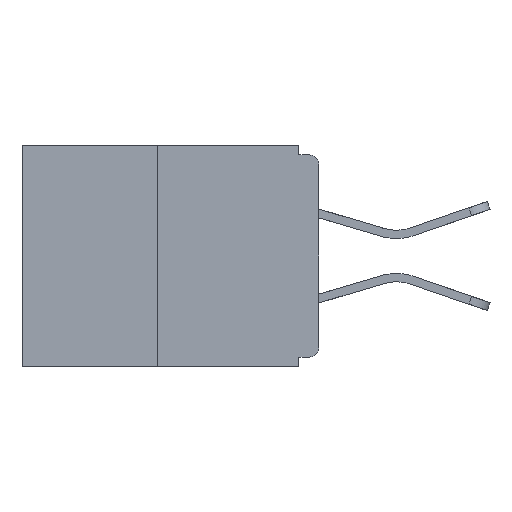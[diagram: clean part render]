
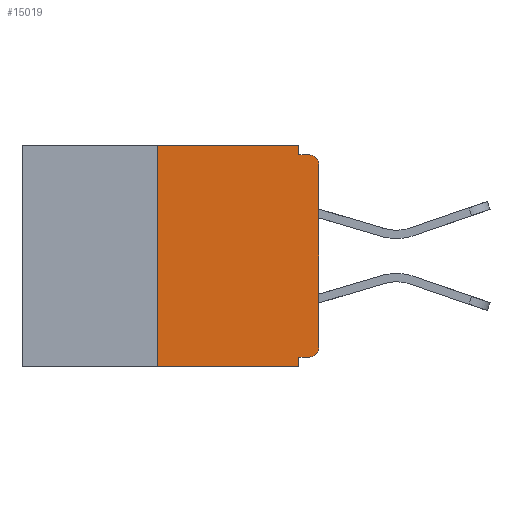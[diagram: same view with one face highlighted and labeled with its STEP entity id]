
A CAD part, left-side view. The second image highlights one B-rep face of the part: STEP entity #15019.
In plain terms, the highlighted planar face has unit normal (-1, 0, 0).
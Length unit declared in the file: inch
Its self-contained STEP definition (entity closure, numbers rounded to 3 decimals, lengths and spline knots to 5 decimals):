
#645 = VERTEX_POINT ( 'NONE', #8346 ) ;
#1054 = VERTEX_POINT ( 'NONE', #18536 ) ;
#2759 = CARTESIAN_POINT ( 'NONE',  ( 0., 0., -0.313 ) ) ;
#2954 = VERTEX_POINT ( 'NONE', #23299 ) ;
#3168 = LINE ( 'NONE', #16092, #10694 ) ;
#3384 = LINE ( 'NONE', #19765, #8680 ) ;
#4042 = ORIENTED_EDGE ( 'NONE', *, *, #25204, .F. ) ;
#4193 = LINE ( 'NONE', #7287, #13943 ) ;
#4215 = EDGE_LOOP ( 'NONE', ( #4042, #20265, #28305, #14607, #9492, #30821, #9199, #12878, #24777, #8813 ) ) ;
#4733 = CARTESIAN_POINT ( 'NONE',  ( 0., 0.015, -0.328 ) ) ;
#4757 = FACE_OUTER_BOUND ( 'NONE', #4215, .T. ) ;
#5252 = CARTESIAN_POINT ( 'NONE',  ( 0., 0., 0. ) ) ;
#5869 = CARTESIAN_POINT ( 'NONE',  ( 0., 0.015, -0.03 ) ) ;
#5882 = CARTESIAN_POINT ( 'NONE',  ( 0., 0.015, -0.313 ) ) ;
#5987 = DIRECTION ( 'NONE',  ( 0., 0., -1. ) ) ;
#6419 = EDGE_CURVE ( 'NONE', #29042, #29580, #3384, .T. ) ;
#6627 = EDGE_CURVE ( 'NONE', #20547, #26070, #18363, .T. ) ;
#6712 = CARTESIAN_POINT ( 'NONE',  ( 0., 0.031, -0.328 ) ) ;
#6923 = CARTESIAN_POINT ( 'NONE',  ( 0., 0.031, 0. ) ) ;
#7287 = CARTESIAN_POINT ( 'NONE',  ( 0., 0.46, -0.343 ) ) ;
#7476 = DIRECTION ( 'NONE',  ( 0., 0., -1. ) ) ;
#8002 = CIRCLE ( 'NONE', #30102, 0.015 ) ;
#8346 = CARTESIAN_POINT ( 'NONE',  ( 0., 0., -0.03 ) ) ;
#8675 = DIRECTION ( 'NONE',  ( 0., 0., 1. ) ) ;
#8680 = VECTOR ( 'NONE', #7476, 39.37008 ) ;
#8813 = ORIENTED_EDGE ( 'NONE', *, *, #6419, .F. ) ;
#8964 = CARTESIAN_POINT ( 'NONE',  ( 0., 0.031, -0.343 ) ) ;
#9162 = EDGE_CURVE ( 'NONE', #29580, #1054, #24224, .T. ) ;
#9199 = ORIENTED_EDGE ( 'NONE', *, *, #20793, .T. ) ;
#9492 = ORIENTED_EDGE ( 'NONE', *, *, #9528, .F. ) ;
#9528 = EDGE_CURVE ( 'NONE', #20547, #20893, #21967, .T. ) ;
#9674 = DIRECTION ( 'NONE',  ( 0., 1., 0. ) ) ;
#10694 = VECTOR ( 'NONE', #18297, 39.37008 ) ;
#10820 = EDGE_CURVE ( 'NONE', #645, #1054, #8002, .T. ) ;
#11066 = VECTOR ( 'NONE', #24237, 39.37008 ) ;
#11077 = VECTOR ( 'NONE', #9674, 39.37008 ) ;
#12878 = ORIENTED_EDGE ( 'NONE', *, *, #10820, .T. ) ;
#13469 = AXIS2_PLACEMENT_3D ( 'NONE', #5882, #15486, #5987 ) ;
#13943 = VECTOR ( 'NONE', #14482, 39.37008 ) ;
#14482 = DIRECTION ( 'NONE',  ( 0., -1., 0. ) ) ;
#14607 = ORIENTED_EDGE ( 'NONE', *, *, #28341, .F. ) ;
#15019 = ADVANCED_FACE ( 'NONE', ( #4757 ), #25930, .F. ) ;
#15097 = DIRECTION ( 'NONE',  ( 0., 0., -1. ) ) ;
#15486 = DIRECTION ( 'NONE',  ( -1., 0., 0. ) ) ;
#15741 = VECTOR ( 'NONE', #15097, 39.37008 ) ;
#16092 = CARTESIAN_POINT ( 'NONE',  ( 0., 0.46, 0. ) ) ;
#17309 = CARTESIAN_POINT ( 'NONE',  ( 0., 0.031, -0.343 ) ) ;
#17439 = LINE ( 'NONE', #5252, #11066 ) ;
#17812 = VECTOR ( 'NONE', #22261, 39.37008 ) ;
#18297 = DIRECTION ( 'NONE',  ( 0., -1., 0. ) ) ;
#18363 = CIRCLE ( 'NONE', #13469, 0.015 ) ;
#18536 = CARTESIAN_POINT ( 'NONE',  ( 0., 0.015, -0.015 ) ) ;
#19765 = CARTESIAN_POINT ( 'NONE',  ( 0., 0.031, 0. ) ) ;
#19865 = DIRECTION ( 'NONE',  ( -1., 0., 0. ) ) ;
#20265 = ORIENTED_EDGE ( 'NONE', *, *, #26957, .F. ) ;
#20547 = VERTEX_POINT ( 'NONE', #4733 ) ;
#20793 = EDGE_CURVE ( 'NONE', #26070, #645, #17439, .T. ) ;
#20893 = VERTEX_POINT ( 'NONE', #6712 ) ;
#21003 = CARTESIAN_POINT ( 'NONE',  ( 0., 0., -0.015 ) ) ;
#21272 = VERTEX_POINT ( 'NONE', #27925 ) ;
#21422 = LINE ( 'NONE', #22169, #27102 ) ;
#21450 = DIRECTION ( 'NONE',  ( 0., 0., -1. ) ) ;
#21711 = CARTESIAN_POINT ( 'NONE',  ( 0., 0., -0.328 ) ) ;
#21967 = LINE ( 'NONE', #21711, #11077 ) ;
#22169 = CARTESIAN_POINT ( 'NONE',  ( 0., 0.25, 0. ) ) ;
#22261 = DIRECTION ( 'NONE',  ( 0., -1., 0. ) ) ;
#23299 = CARTESIAN_POINT ( 'NONE',  ( 0., 0.25, 0. ) ) ;
#24224 = LINE ( 'NONE', #21003, #17812 ) ;
#24237 = DIRECTION ( 'NONE',  ( 0., 0., 1. ) ) ;
#24777 = ORIENTED_EDGE ( 'NONE', *, *, #9162, .F. ) ;
#24980 = DIRECTION ( 'NONE',  ( 0., 0., -1. ) ) ;
#25204 = EDGE_CURVE ( 'NONE', #2954, #29042, #3168, .T. ) ;
#25826 = CARTESIAN_POINT ( 'NONE',  ( 0., 0.46, 0. ) ) ;
#25930 = PLANE ( 'NONE',  #26783 ) ;
#26070 = VERTEX_POINT ( 'NONE', #2759 ) ;
#26783 = AXIS2_PLACEMENT_3D ( 'NONE', #25826, #30866, #21450 ) ;
#26957 = EDGE_CURVE ( 'NONE', #21272, #2954, #21422, .T. ) ;
#27102 = VECTOR ( 'NONE', #8675, 39.37008 ) ;
#27216 = EDGE_CURVE ( 'NONE', #21272, #29847, #4193, .T. ) ;
#27925 = CARTESIAN_POINT ( 'NONE',  ( 0., 0.25, -0.343 ) ) ;
#28305 = ORIENTED_EDGE ( 'NONE', *, *, #27216, .T. ) ;
#28341 = EDGE_CURVE ( 'NONE', #20893, #29847, #30808, .T. ) ;
#29042 = VERTEX_POINT ( 'NONE', #6923 ) ;
#29580 = VERTEX_POINT ( 'NONE', #29842 ) ;
#29842 = CARTESIAN_POINT ( 'NONE',  ( 0., 0.031, -0.015 ) ) ;
#29847 = VERTEX_POINT ( 'NONE', #8964 ) ;
#30102 = AXIS2_PLACEMENT_3D ( 'NONE', #5869, #19865, #24980 ) ;
#30808 = LINE ( 'NONE', #17309, #15741 ) ;
#30821 = ORIENTED_EDGE ( 'NONE', *, *, #6627, .T. ) ;
#30866 = DIRECTION ( 'NONE',  ( 1., 0., 0. ) ) ;
